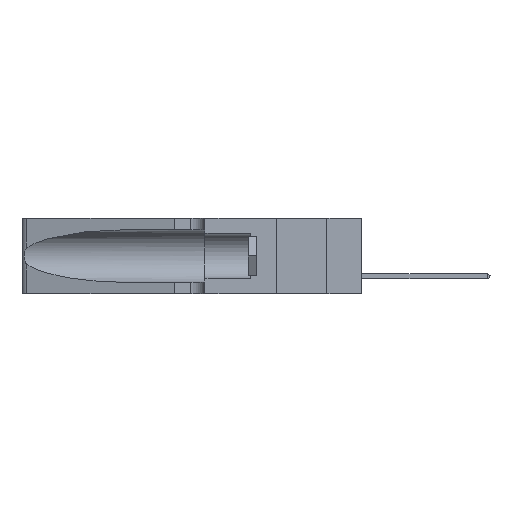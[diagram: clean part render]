
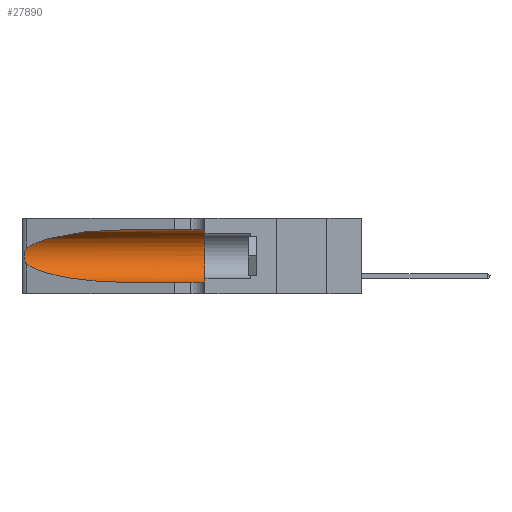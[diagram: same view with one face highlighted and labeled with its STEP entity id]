
A CAD part, left-side view. The second image highlights one B-rep face of the part: STEP entity #27890.
In plain terms, the highlighted cylindrical face has radius 3.308 mm (diameter 6.617 mm), a partial arc.
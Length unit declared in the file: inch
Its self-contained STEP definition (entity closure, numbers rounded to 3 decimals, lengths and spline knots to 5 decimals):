
#1002 = CARTESIAN_POINT ( 'NONE',  ( 0.25639, 1.23184, 0.21858 ) ) ;
#1977 = CARTESIAN_POINT ( 'NONE',  ( 0.2373, 1.15595, 0.08982 ) ) ;
#2419 =( BOUNDED_CURVE ( )  B_SPLINE_CURVE ( 3, ( #39120, #1977, #16144, #30465 ),
 .UNSPECIFIED., .F., .T. ) 
 B_SPLINE_CURVE_WITH_KNOTS ( ( 4, 4 ),
 ( 3.44316, 4.71239 ),
 .UNSPECIFIED. ) 
 CURVE ( )  GEOMETRIC_REPRESENTATION_ITEM ( )  RATIONAL_B_SPLINE_CURVE ( ( 1., 0.87, 0.87, 1. ) ) 
 REPRESENTATION_ITEM ( '' )  );
#4715 = DIRECTION ( 'NONE',  ( 0., -1., 0. ) ) ;
#5114 = VERTEX_POINT ( 'NONE', #20422 ) ;
#5361 = LINE ( 'NONE', #41804, #39193 ) ;
#5562 = CARTESIAN_POINT ( 'NONE',  ( 0.25487, 1.22718, 0.14631 ) ) ;
#7082 = EDGE_CURVE ( 'NONE', #21799, #9671, #31733, .T. ) ;
#7597 = CARTESIAN_POINT ( 'NONE',  ( 0.26075, 1.23896, 0.19203 ) ) ;
#8025 = CARTESIAN_POINT ( 'NONE',  ( 0.26018, 1.23835, 0.19895 ) ) ;
#8524 = EDGE_CURVE ( 'NONE', #26955, #5114, #37937, .T. ) ;
#9671 = VERTEX_POINT ( 'NONE', #13702 ) ;
#10063 = VECTOR ( 'NONE', #21141, 39.37008 ) ;
#11007 = CARTESIAN_POINT ( 'NONE',  ( 0.26017, 1.23833, 0.17102 ) ) ;
#12097 = CARTESIAN_POINT ( 'NONE',  ( 0.25639, 1.23186, 0.15144 ) ) ;
#12168 = CARTESIAN_POINT ( 'NONE',  ( 0.1305, 1.61858, 0.185 ) ) ;
#12337 = ORIENTED_EDGE ( 'NONE', *, *, #7082, .T. ) ;
#13702 = CARTESIAN_POINT ( 'NONE',  ( 0.25487, 1.22718, 0.22369 ) ) ;
#13806 = CARTESIAN_POINT ( 'NONE',  ( 0.1305, 0.35, 0.31525 ) ) ;
#14696 = VERTEX_POINT ( 'NONE', #31305 ) ;
#14764 = AXIS2_PLACEMENT_3D ( 'NONE', #42343, #28487, #32382 ) ;
#16144 = CARTESIAN_POINT ( 'NONE',  ( 0.18966, 0.96281, 0.05475 ) ) ;
#16803 = ORIENTED_EDGE ( 'NONE', *, *, #23997, .T. ) ;
#18015 = EDGE_CURVE ( 'NONE', #21799, #26955, #5361, .T. ) ;
#18606 = DIRECTION ( 'NONE',  ( 0., -1., 0. ) ) ;
#18848 = CARTESIAN_POINT ( 'NONE',  ( 0.25487, 1.22718, 0.22369 ) ) ;
#19926 = ORIENTED_EDGE ( 'NONE', *, *, #34221, .T. ) ;
#20422 = CARTESIAN_POINT ( 'NONE',  ( 0.1305, 0.35, 0.05475 ) ) ;
#21141 = DIRECTION ( 'NONE',  ( 0., -1., 0. ) ) ;
#21799 = VERTEX_POINT ( 'NONE', #30522 ) ;
#22706 = LINE ( 'NONE', #40956, #10063 ) ;
#23997 = EDGE_CURVE ( 'NONE', #9671, #37584, #33139, .T. ) ;
#24114 = ORIENTED_EDGE ( 'NONE', *, *, #8524, .F. ) ;
#25655 = CARTESIAN_POINT ( 'NONE',  ( 0.25555, 1.22993, 0.14849 ) ) ;
#26082 = EDGE_LOOP ( 'NONE', ( #12337, #16803, #19926, #27100, #24114, #39415 ) ) ;
#26257 = CARTESIAN_POINT ( 'NONE',  ( 0.2373, 1.15595, 0.28018 ) ) ;
#26955 = VERTEX_POINT ( 'NONE', #13806 ) ;
#27100 = ORIENTED_EDGE ( 'NONE', *, *, #33882, .T. ) ;
#27257 = AXIS2_PLACEMENT_3D ( 'NONE', #12168, #18606, #36683 ) ;
#27890 = ADVANCED_FACE ( 'NONE', ( #42924 ), #28655, .F. ) ;
#27999 = CARTESIAN_POINT ( 'NONE',  ( 0.25789, 1.23486, 0.15765 ) ) ;
#28297 = CARTESIAN_POINT ( 'NONE',  ( 0.25487, 1.22718, 0.22369 ) ) ;
#28487 = DIRECTION ( 'NONE',  ( 0., 1., 0. ) ) ;
#28655 = CYLINDRICAL_SURFACE ( 'NONE', #27257, 0.13025 ) ;
#29224 = CARTESIAN_POINT ( 'NONE',  ( 0.18966, 0.96281, 0.31525 ) ) ;
#30465 = CARTESIAN_POINT ( 'NONE',  ( 0.1305, 0.72297, 0.05475 ) ) ;
#30522 = CARTESIAN_POINT ( 'NONE',  ( 0.1305, 0.72297, 0.31525 ) ) ;
#31269 = CARTESIAN_POINT ( 'NONE',  ( 0.26075, 1.23896, 0.178 ) ) ;
#31305 = CARTESIAN_POINT ( 'NONE',  ( 0.1305, 0.72297, 0.05475 ) ) ;
#31576 = CARTESIAN_POINT ( 'NONE',  ( 0.25854, 1.2359, 0.20912 ) ) ;
#31733 =( BOUNDED_CURVE ( )  B_SPLINE_CURVE ( 3, ( #35722, #29224, #26257, #18848 ),
 .UNSPECIFIED., .F., .T. ) 
 B_SPLINE_CURVE_WITH_KNOTS ( ( 4, 4 ),
 ( 1.5708, 2.84003 ),
 .UNSPECIFIED. ) 
 CURVE ( )  GEOMETRIC_REPRESENTATION_ITEM ( )  RATIONAL_B_SPLINE_CURVE ( ( 1., 0.87, 0.87, 1. ) ) 
 REPRESENTATION_ITEM ( '' )  );
#32382 = DIRECTION ( 'NONE',  ( 0., 0., 1. ) ) ;
#33139 = B_SPLINE_CURVE_WITH_KNOTS ( 'NONE', 3,
 ( #28297, #41708, #1002, #34968, #31576, #8025, #7597, #31269, #11007, #38031, #27999, #12097, #25655, #5562 ),
 .UNSPECIFIED., .F., .F.,
 ( 4, 2, 2, 2, 2, 2, 4 ),
 ( 0., 0.00027, 0.00053, 0.00107, 0.0016, 0.00187, 0.00214 ),
 .UNSPECIFIED. ) ;
#33882 = EDGE_CURVE ( 'NONE', #14696, #5114, #22706, .T. ) ;
#34221 = EDGE_CURVE ( 'NONE', #37584, #14696, #2419, .T. ) ;
#34968 = CARTESIAN_POINT ( 'NONE',  ( 0.25787, 1.23484, 0.2124 ) ) ;
#35722 = CARTESIAN_POINT ( 'NONE',  ( 0.1305, 0.72297, 0.31525 ) ) ;
#36683 = DIRECTION ( 'NONE',  ( 0., 0., -1. ) ) ;
#37584 = VERTEX_POINT ( 'NONE', #40991 ) ;
#37937 = CIRCLE ( 'NONE', #14764, 0.13025 ) ;
#38031 = CARTESIAN_POINT ( 'NONE',  ( 0.25856, 1.23593, 0.16098 ) ) ;
#39120 = CARTESIAN_POINT ( 'NONE',  ( 0.25487, 1.22718, 0.14631 ) ) ;
#39193 = VECTOR ( 'NONE', #4715, 39.37008 ) ;
#39415 = ORIENTED_EDGE ( 'NONE', *, *, #18015, .F. ) ;
#40956 = CARTESIAN_POINT ( 'NONE',  ( 0.1305, 1.61858, 0.05475 ) ) ;
#40991 = CARTESIAN_POINT ( 'NONE',  ( 0.25487, 1.22718, 0.14631 ) ) ;
#41708 = CARTESIAN_POINT ( 'NONE',  ( 0.25555, 1.22994, 0.2215 ) ) ;
#41804 = CARTESIAN_POINT ( 'NONE',  ( 0.1305, 1.61858, 0.31525 ) ) ;
#42343 = CARTESIAN_POINT ( 'NONE',  ( 0.1305, 0.35, 0.185 ) ) ;
#42924 = FACE_OUTER_BOUND ( 'NONE', #26082, .T. ) ;
